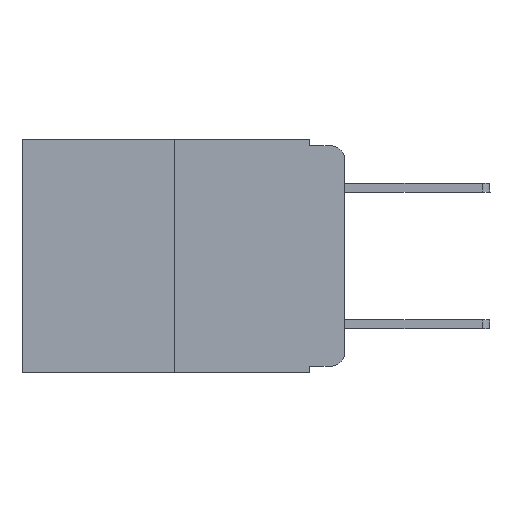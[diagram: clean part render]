
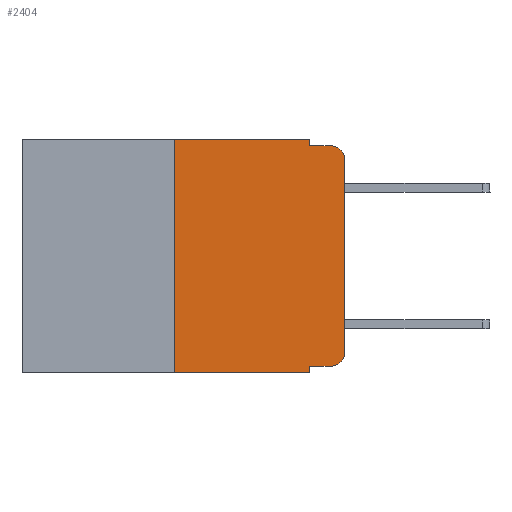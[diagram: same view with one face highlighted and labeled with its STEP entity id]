
A CAD part, left-side view. The second image highlights one B-rep face of the part: STEP entity #2404.
In plain terms, the highlighted planar face has unit normal (-1, 0, 0).
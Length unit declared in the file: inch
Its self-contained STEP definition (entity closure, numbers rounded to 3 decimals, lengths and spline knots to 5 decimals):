
#83 = CARTESIAN_POINT ( 'NONE',  ( 0., 0.051, -0.333 ) ) ;
#217 = ORIENTED_EDGE ( 'NONE', *, *, #8543, .T. ) ;
#257 = CARTESIAN_POINT ( 'NONE',  ( 0., 0.02, -0.03 ) ) ;
#278 = AXIS2_PLACEMENT_3D ( 'NONE', #257, #10226, #2451 ) ;
#304 = VECTOR ( 'NONE', #12183, 39.37008 ) ;
#307 = VECTOR ( 'NONE', #2684, 39.37008 ) ;
#374 = EDGE_CURVE ( 'NONE', #1430, #11171, #8096, .T. ) ;
#700 = CARTESIAN_POINT ( 'NONE',  ( 0., 0.051, -0.343 ) ) ;
#852 = LINE ( 'NONE', #11509, #2702 ) ;
#934 = EDGE_CURVE ( 'NONE', #11131, #11171, #8225, .T. ) ;
#1109 = AXIS2_PLACEMENT_3D ( 'NONE', #5420, #10215, #7440 ) ;
#1379 = VERTEX_POINT ( 'NONE', #7247 ) ;
#1430 = VERTEX_POINT ( 'NONE', #10409 ) ;
#1526 = CARTESIAN_POINT ( 'NONE',  ( 0., 0.051, 0. ) ) ;
#1635 = VERTEX_POINT ( 'NONE', #10692 ) ;
#1757 = DIRECTION ( 'NONE',  ( 0., -1., 0. ) ) ;
#1773 = CARTESIAN_POINT ( 'NONE',  ( 0., 0.051, -0.333 ) ) ;
#1851 = DIRECTION ( 'NONE',  ( 1., 0., 0. ) ) ;
#1983 = PLANE ( 'NONE',  #4320 ) ;
#2149 = VECTOR ( 'NONE', #9649, 39.37008 ) ;
#2404 = ADVANCED_FACE ( 'NONE', ( #7838 ), #1983, .F. ) ;
#2451 = DIRECTION ( 'NONE',  ( 0., 0., -1. ) ) ;
#2577 = VERTEX_POINT ( 'NONE', #11095 ) ;
#2578 = EDGE_CURVE ( 'NONE', #2577, #11222, #3319, .T. ) ;
#2638 = LINE ( 'NONE', #8501, #3437 ) ;
#2684 = DIRECTION ( 'NONE',  ( 0., 0., -1. ) ) ;
#2702 = VECTOR ( 'NONE', #1757, 39.37008 ) ;
#3042 = CARTESIAN_POINT ( 'NONE',  ( 0., 0.473, 0. ) ) ;
#3164 = EDGE_CURVE ( 'NONE', #1430, #1379, #2638, .T. ) ;
#3183 = EDGE_CURVE ( 'NONE', #1379, #1635, #12336, .T. ) ;
#3319 = CIRCLE ( 'NONE', #278, 0.02 ) ;
#3380 = ORIENTED_EDGE ( 'NONE', *, *, #2578, .T. ) ;
#3437 = VECTOR ( 'NONE', #3712, 39.37008 ) ;
#3546 = CARTESIAN_POINT ( 'NONE',  ( 0., 0.02, -0.01 ) ) ;
#3572 = VERTEX_POINT ( 'NONE', #4514 ) ;
#3651 = DIRECTION ( 'NONE',  ( 0., -1., 0. ) ) ;
#3712 = DIRECTION ( 'NONE',  ( 0., 0., 1. ) ) ;
#3820 = DIRECTION ( 'NONE',  ( 0., 0., -1. ) ) ;
#4006 = DIRECTION ( 'NONE',  ( 0., -1., 0. ) ) ;
#4252 = ORIENTED_EDGE ( 'NONE', *, *, #12218, .T. ) ;
#4320 = AXIS2_PLACEMENT_3D ( 'NONE', #3042, #1851, #3820 ) ;
#4496 = CARTESIAN_POINT ( 'NONE',  ( 0., 0.02, -0.333 ) ) ;
#4514 = CARTESIAN_POINT ( 'NONE',  ( 0., 0., -0.313 ) ) ;
#4522 = LINE ( 'NONE', #11208, #307 ) ;
#4854 = ORIENTED_EDGE ( 'NONE', *, *, #3183, .F. ) ;
#5226 = ORIENTED_EDGE ( 'NONE', *, *, #12031, .F. ) ;
#5420 = CARTESIAN_POINT ( 'NONE',  ( 0., 0.02, -0.313 ) ) ;
#5795 = CARTESIAN_POINT ( 'NONE',  ( 0., 0., 0. ) ) ;
#5825 = EDGE_LOOP ( 'NONE', ( #217, #3380, #9924, #5226, #4854, #6001, #7150, #9532, #4252, #7670 ) ) ;
#5882 = LINE ( 'NONE', #83, #11157 ) ;
#6001 = ORIENTED_EDGE ( 'NONE', *, *, #3164, .F. ) ;
#6497 = CARTESIAN_POINT ( 'NONE',  ( 0., 0.051, -0.01 ) ) ;
#6756 = CIRCLE ( 'NONE', #1109, 0.02 ) ;
#7150 = ORIENTED_EDGE ( 'NONE', *, *, #374, .T. ) ;
#7247 = CARTESIAN_POINT ( 'NONE',  ( 0., 0.25, 0. ) ) ;
#7440 = DIRECTION ( 'NONE',  ( 0., 0., -1. ) ) ;
#7670 = ORIENTED_EDGE ( 'NONE', *, *, #11630, .T. ) ;
#7838 = FACE_OUTER_BOUND ( 'NONE', #5825, .T. ) ;
#8096 = LINE ( 'NONE', #11938, #11395 ) ;
#8225 = LINE ( 'NONE', #1526, #304 ) ;
#8268 = VECTOR ( 'NONE', #3651, 39.37008 ) ;
#8501 = CARTESIAN_POINT ( 'NONE',  ( 0., 0.25, 0. ) ) ;
#8543 = EDGE_CURVE ( 'NONE', #3572, #2577, #12294, .T. ) ;
#9116 = DIRECTION ( 'NONE',  ( 0., -1., 0. ) ) ;
#9197 = VERTEX_POINT ( 'NONE', #4496 ) ;
#9322 = CARTESIAN_POINT ( 'NONE',  ( 0., 0.473, 0. ) ) ;
#9532 = ORIENTED_EDGE ( 'NONE', *, *, #934, .F. ) ;
#9649 = DIRECTION ( 'NONE',  ( 0., 0., 1. ) ) ;
#9924 = ORIENTED_EDGE ( 'NONE', *, *, #10172, .F. ) ;
#10172 = EDGE_CURVE ( 'NONE', #11562, #11222, #852, .T. ) ;
#10215 = DIRECTION ( 'NONE',  ( -1., 0., 0. ) ) ;
#10226 = DIRECTION ( 'NONE',  ( -1., 0., 0. ) ) ;
#10409 = CARTESIAN_POINT ( 'NONE',  ( 0., 0.25, -0.343 ) ) ;
#10692 = CARTESIAN_POINT ( 'NONE',  ( 0., 0.051, 0. ) ) ;
#11095 = CARTESIAN_POINT ( 'NONE',  ( 0., 0., -0.03 ) ) ;
#11131 = VERTEX_POINT ( 'NONE', #1773 ) ;
#11157 = VECTOR ( 'NONE', #4006, 39.37008 ) ;
#11171 = VERTEX_POINT ( 'NONE', #700 ) ;
#11208 = CARTESIAN_POINT ( 'NONE',  ( 0., 0.051, 0. ) ) ;
#11222 = VERTEX_POINT ( 'NONE', #3546 ) ;
#11395 = VECTOR ( 'NONE', #9116, 39.37008 ) ;
#11509 = CARTESIAN_POINT ( 'NONE',  ( 0., 0.051, -0.01 ) ) ;
#11562 = VERTEX_POINT ( 'NONE', #6497 ) ;
#11630 = EDGE_CURVE ( 'NONE', #9197, #3572, #6756, .T. ) ;
#11938 = CARTESIAN_POINT ( 'NONE',  ( 0., 0.473, -0.343 ) ) ;
#12031 = EDGE_CURVE ( 'NONE', #1635, #11562, #4522, .T. ) ;
#12183 = DIRECTION ( 'NONE',  ( 0., 0., -1. ) ) ;
#12218 = EDGE_CURVE ( 'NONE', #11131, #9197, #5882, .T. ) ;
#12294 = LINE ( 'NONE', #5795, #2149 ) ;
#12336 = LINE ( 'NONE', #9322, #8268 ) ;
